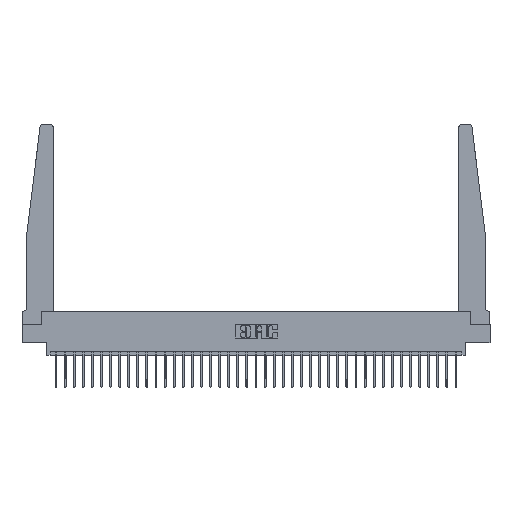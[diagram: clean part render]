
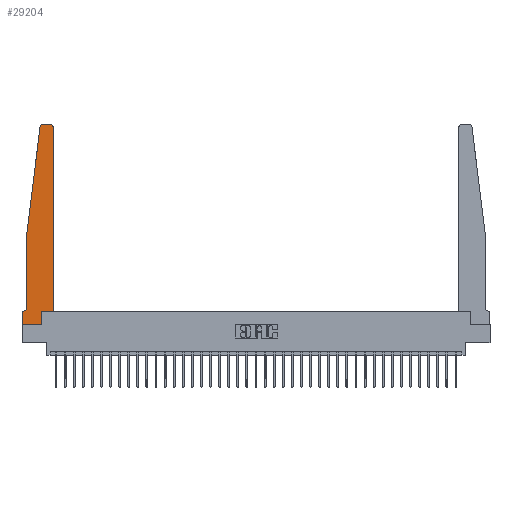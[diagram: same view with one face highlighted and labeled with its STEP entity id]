
A CAD part, top view. The second image highlights one B-rep face of the part: STEP entity #29204.
In plain terms, the highlighted planar face has unit normal (0, 0, 1).
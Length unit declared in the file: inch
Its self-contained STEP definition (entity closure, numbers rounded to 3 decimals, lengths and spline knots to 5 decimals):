
#159 = VERTEX_POINT ( 'NONE', #19447 ) ;
#332 = ORIENTED_EDGE ( 'NONE', *, *, #32586, .T. ) ;
#497 = VERTEX_POINT ( 'NONE', #13538 ) ;
#831 = ORIENTED_EDGE ( 'NONE', *, *, #10897, .T. ) ;
#1015 = VECTOR ( 'NONE', #13367, 39.37008 ) ;
#1502 = VERTEX_POINT ( 'NONE', #21186 ) ;
#1991 = EDGE_CURVE ( 'NONE', #18696, #16167, #13524, .T. ) ;
#2045 = AXIS2_PLACEMENT_3D ( 'NONE', #31968, #10435, #18409 ) ;
#2285 = EDGE_CURVE ( 'NONE', #497, #11838, #4633, .T. ) ;
#2517 = CARTESIAN_POINT ( 'NONE',  ( 0.015, 0.1875, 0.37 ) ) ;
#2889 = AXIS2_PLACEMENT_3D ( 'NONE', #22569, #3303, #30070 ) ;
#3303 = DIRECTION ( 'NONE',  ( 0., 0., 1. ) ) ;
#4451 = CIRCLE ( 'NONE', #17767, 0.05 ) ;
#4633 = LINE ( 'NONE', #15064, #4882 ) ;
#4696 = VERTEX_POINT ( 'NONE', #7291 ) ;
#4784 = VECTOR ( 'NONE', #26434, 39.37008 ) ;
#4872 = DIRECTION ( 'NONE',  ( 0., 1., 0. ) ) ;
#4882 = VECTOR ( 'NONE', #12451, 39.37008 ) ;
#4937 = ORIENTED_EDGE ( 'NONE', *, *, #9763, .T. ) ;
#4969 = EDGE_CURVE ( 'NONE', #159, #21755, #18058, .T. ) ;
#5367 = LINE ( 'NONE', #31631, #17736 ) ;
#5484 = DIRECTION ( 'NONE',  ( 0., -1., 0. ) ) ;
#6007 = DIRECTION ( 'NONE',  ( -1., 0., 0. ) ) ;
#7151 = ORIENTED_EDGE ( 'NONE', *, *, #2285, .T. ) ;
#7291 = CARTESIAN_POINT ( 'NONE',  ( 0., 0., 0.37 ) ) ;
#7583 = VECTOR ( 'NONE', #5484, 39.37008 ) ;
#8085 = LINE ( 'NONE', #18683, #7583 ) ;
#8768 = VECTOR ( 'NONE', #23753, 39.37008 ) ;
#9551 = CIRCLE ( 'NONE', #2889, 0.03 ) ;
#9589 = ORIENTED_EDGE ( 'NONE', *, *, #25526, .T. ) ;
#9763 = EDGE_CURVE ( 'NONE', #11838, #12884, #32036, .T. ) ;
#10274 = ORIENTED_EDGE ( 'NONE', *, *, #10509, .T. ) ;
#10414 = DIRECTION ( 'NONE',  ( 0., 0., -1. ) ) ;
#10435 = DIRECTION ( 'NONE',  ( 0., 0., 1. ) ) ;
#10509 = EDGE_CURVE ( 'NONE', #16167, #159, #26608, .T. ) ;
#10897 = EDGE_CURVE ( 'NONE', #32264, #4696, #5367, .T. ) ;
#11223 = LINE ( 'NONE', #19027, #24249 ) ;
#11838 = VERTEX_POINT ( 'NONE', #31554 ) ;
#12451 = DIRECTION ( 'NONE',  ( -1., 0., 0. ) ) ;
#12884 = VERTEX_POINT ( 'NONE', #16643 ) ;
#13338 = AXIS2_PLACEMENT_3D ( 'NONE', #15807, #23244, #26017 ) ;
#13352 = CARTESIAN_POINT ( 'NONE',  ( 0.2605, 0.18, 0.37 ) ) ;
#13367 = DIRECTION ( 'NONE',  ( 1., 0., 0. ) ) ;
#13423 = CARTESIAN_POINT ( 'NONE',  ( 0.425, 0.18, 0.37 ) ) ;
#13505 = VERTEX_POINT ( 'NONE', #26775 ) ;
#13524 = LINE ( 'NONE', #13352, #8768 ) ;
#13538 = CARTESIAN_POINT ( 'NONE',  ( 0.395, 2.75, 0.37 ) ) ;
#13939 = CARTESIAN_POINT ( 'NONE',  ( 0., 0.1875, 0.37 ) ) ;
#14209 = EDGE_LOOP ( 'NONE', ( #7151, #4937, #332, #30757, #24957, #20350, #831, #9589, #19634, #10274, #24449, #29040 ) ) ;
#14369 = EDGE_CURVE ( 'NONE', #21755, #497, #9551, .T. ) ;
#15064 = CARTESIAN_POINT ( 'NONE',  ( 0.25, 2.75, 0.37 ) ) ;
#15465 = FACE_OUTER_BOUND ( 'NONE', #14209, .T. ) ;
#15677 = LINE ( 'NONE', #21190, #26215 ) ;
#15807 = CARTESIAN_POINT ( 'NONE',  ( 0., 0.1875, 0.37 ) ) ;
#16143 = PLANE ( 'NONE',  #13338 ) ;
#16167 = VERTEX_POINT ( 'NONE', #20084 ) ;
#16643 = CARTESIAN_POINT ( 'NONE',  ( 0.24675, 2.72367, 0.37 ) ) ;
#17736 = VECTOR ( 'NONE', #18916, 39.37008 ) ;
#17767 = AXIS2_PLACEMENT_3D ( 'NONE', #26535, #10414, #20969 ) ;
#18058 = LINE ( 'NONE', #18232, #29790 ) ;
#18232 = CARTESIAN_POINT ( 'NONE',  ( 0.425, 0.18, 0.37 ) ) ;
#18409 = DIRECTION ( 'NONE',  ( 1., 0., 0. ) ) ;
#18683 = CARTESIAN_POINT ( 'NONE',  ( 0.065, 1.25, 0.37 ) ) ;
#18696 = VERTEX_POINT ( 'NONE', #21562 ) ;
#18916 = DIRECTION ( 'NONE',  ( 0., -1., 0. ) ) ;
#19027 = CARTESIAN_POINT ( 'NONE',  ( 0.065, 0.1875, 0.37 ) ) ;
#19071 = CARTESIAN_POINT ( 'NONE',  ( 0., 0., 0.37 ) ) ;
#19247 = LINE ( 'NONE', #19071, #1015 ) ;
#19447 = CARTESIAN_POINT ( 'NONE',  ( 0.425, 0.18, 0.37 ) ) ;
#19634 = ORIENTED_EDGE ( 'NONE', *, *, #1991, .T. ) ;
#20084 = CARTESIAN_POINT ( 'NONE',  ( 0.2605, 0.18, 0.37 ) ) ;
#20350 = ORIENTED_EDGE ( 'NONE', *, *, #24039, .T. ) ;
#20969 = DIRECTION ( 'NONE',  ( -1., 0., 0. ) ) ;
#21186 = CARTESIAN_POINT ( 'NONE',  ( 0.065, 0.2375, 0.37 ) ) ;
#21190 = CARTESIAN_POINT ( 'NONE',  ( 0.065, 1.25, 0.37 ) ) ;
#21562 = CARTESIAN_POINT ( 'NONE',  ( 0.2605, 0., 0.37 ) ) ;
#21755 = VERTEX_POINT ( 'NONE', #30240 ) ;
#22539 = VERTEX_POINT ( 'NONE', #2517 ) ;
#22569 = CARTESIAN_POINT ( 'NONE',  ( 0.395, 2.72, 0.37 ) ) ;
#22665 = EDGE_CURVE ( 'NONE', #13505, #1502, #8085, .T. ) ;
#23244 = DIRECTION ( 'NONE',  ( 0., 0., 1. ) ) ;
#23753 = DIRECTION ( 'NONE',  ( 0., 1., 0. ) ) ;
#24039 = EDGE_CURVE ( 'NONE', #22539, #32264, #11223, .T. ) ;
#24249 = VECTOR ( 'NONE', #6007, 39.37008 ) ;
#24449 = ORIENTED_EDGE ( 'NONE', *, *, #4969, .T. ) ;
#24957 = ORIENTED_EDGE ( 'NONE', *, *, #29302, .T. ) ;
#25526 = EDGE_CURVE ( 'NONE', #4696, #18696, #19247, .T. ) ;
#26017 = DIRECTION ( 'NONE',  ( 1., 0., 0. ) ) ;
#26215 = VECTOR ( 'NONE', #28693, 39.37008 ) ;
#26434 = DIRECTION ( 'NONE',  ( 1., 0., 0. ) ) ;
#26535 = CARTESIAN_POINT ( 'NONE',  ( 0.015, 0.2375, 0.37 ) ) ;
#26608 = LINE ( 'NONE', #13423, #4784 ) ;
#26775 = CARTESIAN_POINT ( 'NONE',  ( 0.065, 1.25, 0.37 ) ) ;
#28693 = DIRECTION ( 'NONE',  ( -0.122, -0.992, 0. ) ) ;
#29040 = ORIENTED_EDGE ( 'NONE', *, *, #14369, .T. ) ;
#29204 = ADVANCED_FACE ( 'NONE', ( #15465 ), #16143, .T. ) ;
#29302 = EDGE_CURVE ( 'NONE', #1502, #22539, #4451, .T. ) ;
#29790 = VECTOR ( 'NONE', #4872, 39.37008 ) ;
#30070 = DIRECTION ( 'NONE',  ( 1., 0., 0. ) ) ;
#30240 = CARTESIAN_POINT ( 'NONE',  ( 0.425, 2.72, 0.37 ) ) ;
#30757 = ORIENTED_EDGE ( 'NONE', *, *, #22665, .T. ) ;
#31554 = CARTESIAN_POINT ( 'NONE',  ( 0.27653, 2.75, 0.37 ) ) ;
#31631 = CARTESIAN_POINT ( 'NONE',  ( 0., 0., 0.37 ) ) ;
#31968 = CARTESIAN_POINT ( 'NONE',  ( 0.27653, 2.72, 0.37 ) ) ;
#32036 = CIRCLE ( 'NONE', #2045, 0.03 ) ;
#32264 = VERTEX_POINT ( 'NONE', #13939 ) ;
#32586 = EDGE_CURVE ( 'NONE', #12884, #13505, #15677, .T. ) ;
